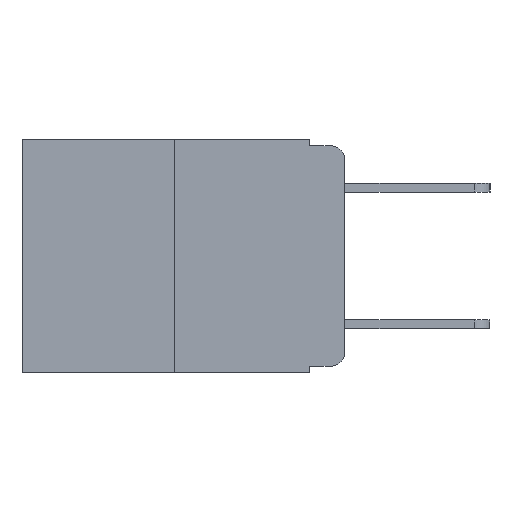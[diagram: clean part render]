
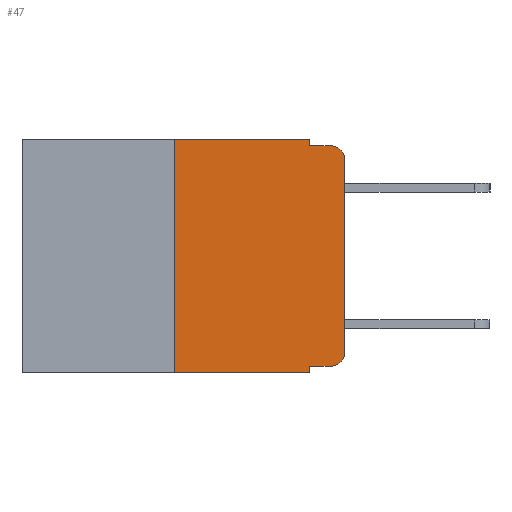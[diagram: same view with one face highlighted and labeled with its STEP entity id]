
A CAD part, left-side view. The second image highlights one B-rep face of the part: STEP entity #47.
In plain terms, the highlighted planar face has unit normal (-1, 0, 0).
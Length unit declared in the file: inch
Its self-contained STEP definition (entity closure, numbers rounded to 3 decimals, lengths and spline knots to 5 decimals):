
#47 = ADVANCED_FACE ( 'NONE', ( #11405 ), #11097, .F. ) ;
#210 = CARTESIAN_POINT ( 'NONE',  ( 0., 0.25, 0. ) ) ;
#437 = VERTEX_POINT ( 'NONE', #11034 ) ;
#499 = DIRECTION ( 'NONE',  ( 0., 0., -1. ) ) ;
#539 = DIRECTION ( 'NONE',  ( 0., 0., -1. ) ) ;
#624 = CARTESIAN_POINT ( 'NONE',  ( 0., 0.051, 0. ) ) ;
#723 = EDGE_CURVE ( 'NONE', #7065, #437, #5482, .T. ) ;
#887 = VECTOR ( 'NONE', #1485, 39.37008 ) ;
#970 = LINE ( 'NONE', #2993, #3599 ) ;
#1098 = VERTEX_POINT ( 'NONE', #1687 ) ;
#1153 = DIRECTION ( 'NONE',  ( 0., -1., 0. ) ) ;
#1423 = EDGE_CURVE ( 'NONE', #2783, #9302, #4829, .T. ) ;
#1485 = DIRECTION ( 'NONE',  ( 0., -1., 0. ) ) ;
#1654 = VERTEX_POINT ( 'NONE', #9623 ) ;
#1659 = DIRECTION ( 'NONE',  ( 0., 0., -1. ) ) ;
#1687 = CARTESIAN_POINT ( 'NONE',  ( 0., 0.051, -0.343 ) ) ;
#2104 = DIRECTION ( 'NONE',  ( 1., 0., 0. ) ) ;
#2542 = CARTESIAN_POINT ( 'NONE',  ( 0., 0.473, 0. ) ) ;
#2741 = EDGE_CURVE ( 'NONE', #9302, #7065, #970, .T. ) ;
#2783 = VERTEX_POINT ( 'NONE', #9643 ) ;
#2953 = VECTOR ( 'NONE', #7958, 39.37008 ) ;
#2993 = CARTESIAN_POINT ( 'NONE',  ( 0., 0.051, 0. ) ) ;
#3049 = CARTESIAN_POINT ( 'NONE',  ( 0., 0., 0. ) ) ;
#3096 = VERTEX_POINT ( 'NONE', #3538 ) ;
#3538 = CARTESIAN_POINT ( 'NONE',  ( 0., 0.02, -0.333 ) ) ;
#3599 = VECTOR ( 'NONE', #9601, 39.37008 ) ;
#4462 = DIRECTION ( 'NONE',  ( 0., -1., 0. ) ) ;
#4528 = AXIS2_PLACEMENT_3D ( 'NONE', #11820, #6350, #499 ) ;
#4643 = CARTESIAN_POINT ( 'NONE',  ( 0., 0.051, -0.333 ) ) ;
#4659 = CIRCLE ( 'NONE', #9027, 0.02 ) ;
#4738 = EDGE_LOOP ( 'NONE', ( #7404, #9565, #10409, #8835, #12099, #11840, #10294, #6568, #4894, #11659 ) ) ;
#4829 = LINE ( 'NONE', #2542, #11925 ) ;
#4894 = ORIENTED_EDGE ( 'NONE', *, *, #7736, .T. ) ;
#5020 = CARTESIAN_POINT ( 'NONE',  ( 0., 0.051, -0.01 ) ) ;
#5482 = LINE ( 'NONE', #5020, #887 ) ;
#5931 = VERTEX_POINT ( 'NONE', #8993 ) ;
#6332 = LINE ( 'NONE', #3049, #10639 ) ;
#6350 = DIRECTION ( 'NONE',  ( -1., 0., 0. ) ) ;
#6392 = DIRECTION ( 'NONE',  ( -1., 0., 0. ) ) ;
#6568 = ORIENTED_EDGE ( 'NONE', *, *, #10814, .F. ) ;
#6639 = LINE ( 'NONE', #4643, #8489 ) ;
#6686 = VERTEX_POINT ( 'NONE', #10187 ) ;
#7065 = VERTEX_POINT ( 'NONE', #11705 ) ;
#7129 = EDGE_CURVE ( 'NONE', #3096, #6686, #8373, .T. ) ;
#7404 = ORIENTED_EDGE ( 'NONE', *, *, #8892, .T. ) ;
#7736 = EDGE_CURVE ( 'NONE', #5931, #3096, #6639, .T. ) ;
#7893 = AXIS2_PLACEMENT_3D ( 'NONE', #11026, #2104, #10961 ) ;
#7958 = DIRECTION ( 'NONE',  ( 0., 0., 1. ) ) ;
#8017 = LINE ( 'NONE', #210, #2953 ) ;
#8290 = EDGE_CURVE ( 'NONE', #1654, #1098, #12167, .T. ) ;
#8307 = CARTESIAN_POINT ( 'NONE',  ( 0., 0., -0.03 ) ) ;
#8373 = CIRCLE ( 'NONE', #4528, 0.02 ) ;
#8489 = VECTOR ( 'NONE', #9326, 39.37008 ) ;
#8565 = EDGE_CURVE ( 'NONE', #9290, #437, #4659, .T. ) ;
#8835 = ORIENTED_EDGE ( 'NONE', *, *, #2741, .F. ) ;
#8892 = EDGE_CURVE ( 'NONE', #6686, #9290, #6332, .T. ) ;
#8993 = CARTESIAN_POINT ( 'NONE',  ( 0., 0.051, -0.333 ) ) ;
#9027 = AXIS2_PLACEMENT_3D ( 'NONE', #11856, #6392, #539 ) ;
#9029 = LINE ( 'NONE', #624, #11159 ) ;
#9290 = VERTEX_POINT ( 'NONE', #8307 ) ;
#9302 = VERTEX_POINT ( 'NONE', #10156 ) ;
#9326 = DIRECTION ( 'NONE',  ( 0., -1., 0. ) ) ;
#9565 = ORIENTED_EDGE ( 'NONE', *, *, #8565, .T. ) ;
#9601 = DIRECTION ( 'NONE',  ( 0., 0., -1. ) ) ;
#9623 = CARTESIAN_POINT ( 'NONE',  ( 0., 0.25, -0.343 ) ) ;
#9643 = CARTESIAN_POINT ( 'NONE',  ( 0., 0.25, 0. ) ) ;
#9798 = VECTOR ( 'NONE', #1153, 39.37008 ) ;
#10156 = CARTESIAN_POINT ( 'NONE',  ( 0., 0.051, 0. ) ) ;
#10187 = CARTESIAN_POINT ( 'NONE',  ( 0., 0., -0.313 ) ) ;
#10294 = ORIENTED_EDGE ( 'NONE', *, *, #8290, .T. ) ;
#10409 = ORIENTED_EDGE ( 'NONE', *, *, #723, .F. ) ;
#10545 = DIRECTION ( 'NONE',  ( 0., 0., 1. ) ) ;
#10599 = CARTESIAN_POINT ( 'NONE',  ( 0., 0.473, -0.343 ) ) ;
#10639 = VECTOR ( 'NONE', #10545, 39.37008 ) ;
#10814 = EDGE_CURVE ( 'NONE', #5931, #1098, #9029, .T. ) ;
#10961 = DIRECTION ( 'NONE',  ( 0., 0., -1. ) ) ;
#11026 = CARTESIAN_POINT ( 'NONE',  ( 0., 0.473, 0. ) ) ;
#11034 = CARTESIAN_POINT ( 'NONE',  ( 0., 0.02, -0.01 ) ) ;
#11097 = PLANE ( 'NONE',  #7893 ) ;
#11159 = VECTOR ( 'NONE', #1659, 39.37008 ) ;
#11160 = EDGE_CURVE ( 'NONE', #1654, #2783, #8017, .T. ) ;
#11405 = FACE_OUTER_BOUND ( 'NONE', #4738, .T. ) ;
#11659 = ORIENTED_EDGE ( 'NONE', *, *, #7129, .T. ) ;
#11705 = CARTESIAN_POINT ( 'NONE',  ( 0., 0.051, -0.01 ) ) ;
#11820 = CARTESIAN_POINT ( 'NONE',  ( 0., 0.02, -0.313 ) ) ;
#11840 = ORIENTED_EDGE ( 'NONE', *, *, #11160, .F. ) ;
#11856 = CARTESIAN_POINT ( 'NONE',  ( 0., 0.02, -0.03 ) ) ;
#11925 = VECTOR ( 'NONE', #4462, 39.37008 ) ;
#12099 = ORIENTED_EDGE ( 'NONE', *, *, #1423, .F. ) ;
#12167 = LINE ( 'NONE', #10599, #9798 ) ;
